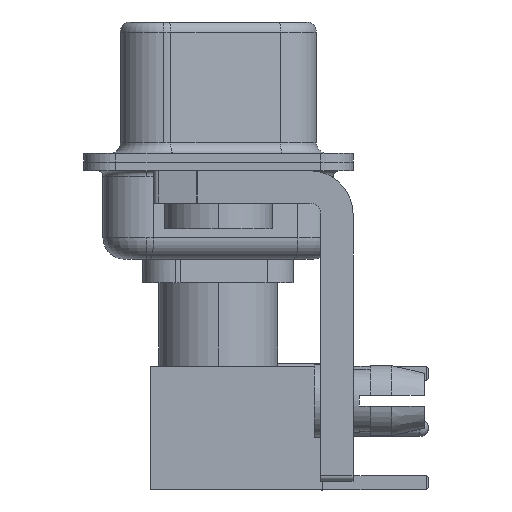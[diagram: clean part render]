
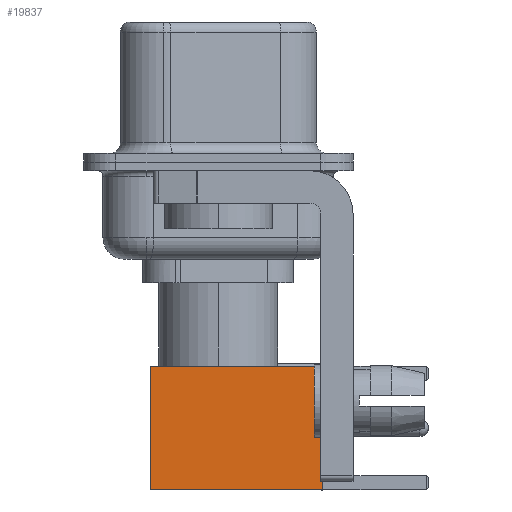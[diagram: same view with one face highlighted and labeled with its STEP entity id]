
A CAD part, left-side view. The second image highlights one B-rep face of the part: STEP entity #19837.
In plain terms, the highlighted face is planar.
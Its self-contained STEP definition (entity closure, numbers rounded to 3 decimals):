
#115 = DIRECTION ( 'NONE',  ( 0., 1., 0. ) ) ;
#1121 = ORIENTED_EDGE ( 'NONE', *, *, #14398, .T. ) ;
#1807 = DIRECTION ( 'NONE',  ( -1., 0., 0. ) ) ;
#2548 = CARTESIAN_POINT ( 'NONE',  ( -2.875, 2.875, 0. ) ) ;
#3325 = VECTOR ( 'NONE', #9366, 1000. ) ;
#3677 = DIRECTION ( 'NONE',  ( -1., 0., 0. ) ) ;
#4150 = VERTEX_POINT ( 'NONE', #12442 ) ;
#4949 = VECTOR ( 'NONE', #6200, 1000. ) ;
#5033 = ORIENTED_EDGE ( 'NONE', *, *, #24052, .F. ) ;
#5909 = LINE ( 'NONE', #22541, #4949 ) ;
#6200 = DIRECTION ( 'NONE',  ( 0., 0., -1. ) ) ;
#7640 = EDGE_CURVE ( 'NONE', #4150, #12500, #27082, .T. ) ;
#9366 = DIRECTION ( 'NONE',  ( 0., 0., -1. ) ) ;
#10909 = VECTOR ( 'NONE', #3677, 1000. ) ;
#11645 = LINE ( 'NONE', #2548, #3325 ) ;
#12017 = VERTEX_POINT ( 'NONE', #24098 ) ;
#12423 = CARTESIAN_POINT ( 'NONE',  ( -2.875, 2.875, 0. ) ) ;
#12442 = CARTESIAN_POINT ( 'NONE',  ( 2.875, 2.875, 0. ) ) ;
#12500 = VERTEX_POINT ( 'NONE', #12423 ) ;
#13440 = DIRECTION ( 'NONE',  ( 0., 0., 1. ) ) ;
#14398 = EDGE_CURVE ( 'NONE', #22028, #4150, #5909, .T. ) ;
#14754 = LINE ( 'NONE', #23958, #10909 ) ;
#14946 = EDGE_LOOP ( 'NONE', ( #1121, #23035, #5033, #28793 ) ) ;
#15074 = CARTESIAN_POINT ( 'NONE',  ( 2.875, 2.875, 8. ) ) ;
#18439 = CARTESIAN_POINT ( 'NONE',  ( 2.875, 2.875, 0. ) ) ;
#19224 = EDGE_CURVE ( 'NONE', #22028, #12017, #14754, .T. ) ;
#19837 = ADVANCED_FACE ( 'NONE', ( #27507 ), #20988, .T. ) ;
#20710 = VECTOR ( 'NONE', #1807, 1000. ) ;
#20988 = PLANE ( 'NONE',  #25427 ) ;
#22028 = VERTEX_POINT ( 'NONE', #15074 ) ;
#22541 = CARTESIAN_POINT ( 'NONE',  ( 2.875, 2.875, 0. ) ) ;
#22819 = CARTESIAN_POINT ( 'NONE',  ( 0., 2.875, 0. ) ) ;
#23035 = ORIENTED_EDGE ( 'NONE', *, *, #7640, .T. ) ;
#23958 = CARTESIAN_POINT ( 'NONE',  ( 0., 2.875, 8. ) ) ;
#24052 = EDGE_CURVE ( 'NONE', #12017, #12500, #11645, .T. ) ;
#24098 = CARTESIAN_POINT ( 'NONE',  ( -2.875, 2.875, 8. ) ) ;
#25427 = AXIS2_PLACEMENT_3D ( 'NONE', #18439, #115, #13440 ) ;
#27082 = LINE ( 'NONE', #22819, #20710 ) ;
#27507 = FACE_OUTER_BOUND ( 'NONE', #14946, .T. ) ;
#28793 = ORIENTED_EDGE ( 'NONE', *, *, #19224, .F. ) ;
